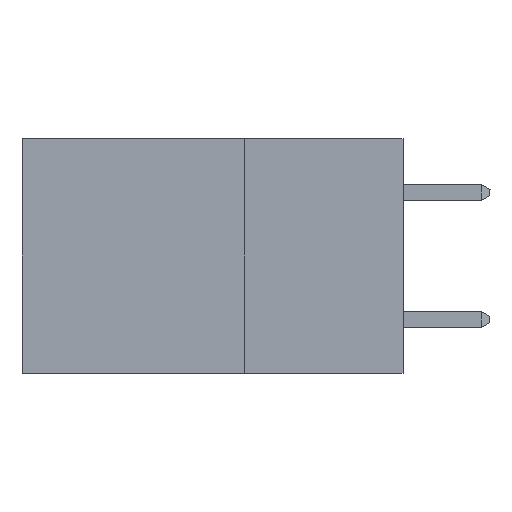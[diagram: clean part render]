
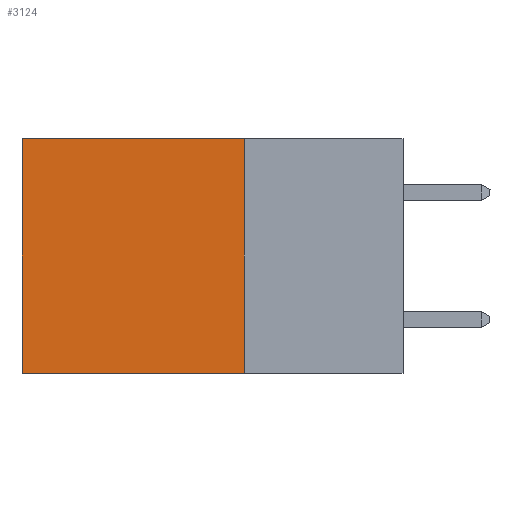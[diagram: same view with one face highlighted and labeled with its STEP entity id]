
A CAD part, left-side view. The second image highlights one B-rep face of the part: STEP entity #3124.
In plain terms, the highlighted planar face has unit normal (-1, 0, 0).
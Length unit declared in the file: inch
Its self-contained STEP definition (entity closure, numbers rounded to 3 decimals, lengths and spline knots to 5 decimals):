
#449 = CARTESIAN_POINT ( 'NONE',  ( 0.2875, 0.25, 0. ) ) ;
#791 = AXIS2_PLACEMENT_3D ( 'NONE', #449, #15874, #4568 ) ;
#1375 = EDGE_CURVE ( 'NONE', #14115, #23486, #21120, .T. ) ;
#1445 = CARTESIAN_POINT ( 'NONE',  ( 0.2875, 0.6, 0. ) ) ;
#2266 = CARTESIAN_POINT ( 'NONE',  ( 0.2875, 0.25, 0. ) ) ;
#2612 = PLANE ( 'NONE',  #791 ) ;
#2866 = CARTESIAN_POINT ( 'NONE',  ( 0.2875, 0.25, 0. ) ) ;
#2912 = ORIENTED_EDGE ( 'NONE', *, *, #5065, .F. ) ;
#3124 = ADVANCED_FACE ( 'NONE', ( #18974 ), #2612, .F. ) ;
#3140 = VECTOR ( 'NONE', #7827, 39.37008 ) ;
#3407 = ORIENTED_EDGE ( 'NONE', *, *, #6328, .F. ) ;
#4568 = DIRECTION ( 'NONE',  ( 0., 0., -1. ) ) ;
#5046 = ORIENTED_EDGE ( 'NONE', *, *, #1375, .T. ) ;
#5065 = EDGE_CURVE ( 'NONE', #14115, #6051, #6491, .T. ) ;
#5950 = CARTESIAN_POINT ( 'NONE',  ( 0.2875, 0.25, -0.37 ) ) ;
#6051 = VERTEX_POINT ( 'NONE', #16530 ) ;
#6328 = EDGE_CURVE ( 'NONE', #6051, #24411, #18239, .T. ) ;
#6339 = DIRECTION ( 'NONE',  ( 0., 0., -1. ) ) ;
#6491 = LINE ( 'NONE', #2266, #17130 ) ;
#7827 = DIRECTION ( 'NONE',  ( 0., 1., 0. ) ) ;
#8707 = LINE ( 'NONE', #10035, #18180 ) ;
#10035 = CARTESIAN_POINT ( 'NONE',  ( 0.2875, 0.6, 0. ) ) ;
#14074 = ORIENTED_EDGE ( 'NONE', *, *, #21297, .T. ) ;
#14115 = VERTEX_POINT ( 'NONE', #2866 ) ;
#15874 = DIRECTION ( 'NONE',  ( 1., 0., 0. ) ) ;
#16530 = CARTESIAN_POINT ( 'NONE',  ( 0.2875, 0.25, -0.37 ) ) ;
#17130 = VECTOR ( 'NONE', #17435, 39.37008 ) ;
#17435 = DIRECTION ( 'NONE',  ( 0., 0., -1. ) ) ;
#18180 = VECTOR ( 'NONE', #6339, 39.37008 ) ;
#18239 = LINE ( 'NONE', #5950, #3140 ) ;
#18974 = FACE_OUTER_BOUND ( 'NONE', #19252, .T. ) ;
#19252 = EDGE_LOOP ( 'NONE', ( #14074, #3407, #2912, #5046 ) ) ;
#20518 = VECTOR ( 'NONE', #20963, 39.37008 ) ;
#20963 = DIRECTION ( 'NONE',  ( 0., 1., 0. ) ) ;
#21120 = LINE ( 'NONE', #21740, #20518 ) ;
#21297 = EDGE_CURVE ( 'NONE', #23486, #24411, #8707, .T. ) ;
#21740 = CARTESIAN_POINT ( 'NONE',  ( 0.2875, 0.25, 0. ) ) ;
#22208 = CARTESIAN_POINT ( 'NONE',  ( 0.2875, 0.6, -0.37 ) ) ;
#23486 = VERTEX_POINT ( 'NONE', #1445 ) ;
#24411 = VERTEX_POINT ( 'NONE', #22208 ) ;
